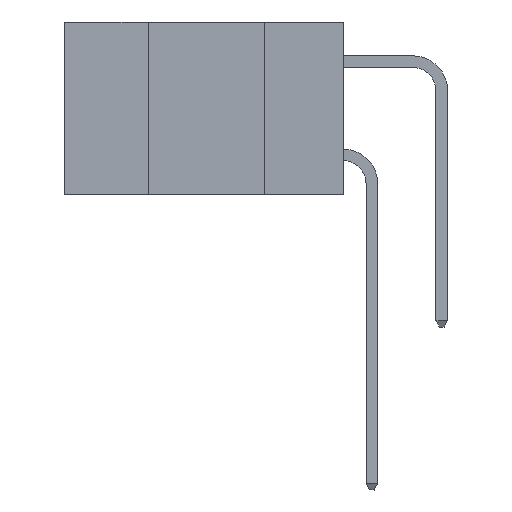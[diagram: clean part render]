
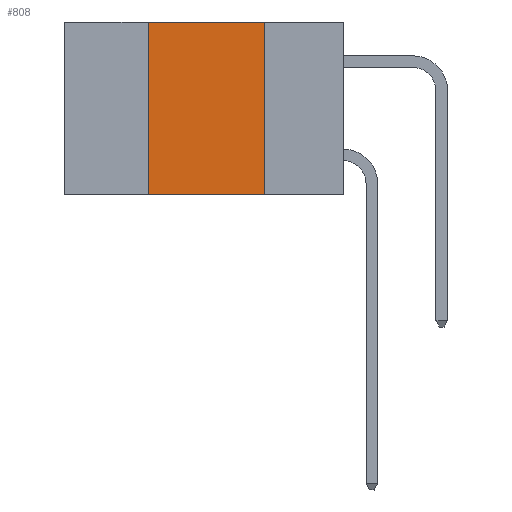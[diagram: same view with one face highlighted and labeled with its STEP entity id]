
A CAD part, left-side view. The second image highlights one B-rep face of the part: STEP entity #808.
In plain terms, the highlighted planar face has unit normal (-1, 0, 0).
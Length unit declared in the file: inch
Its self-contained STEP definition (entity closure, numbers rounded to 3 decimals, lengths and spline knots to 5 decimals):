
#54 = EDGE_CURVE ( 'NONE', #7547, #682, #2304, .T. ) ;
#215 = EDGE_CURVE ( 'NONE', #682, #5198, #5737, .T. ) ;
#250 = CARTESIAN_POINT ( 'NONE',  ( 0., 0.17, -0.37 ) ) ;
#503 = AXIS2_PLACEMENT_3D ( 'NONE', #5268, #9201, #7152 ) ;
#682 = VERTEX_POINT ( 'NONE', #9652 ) ;
#808 = ADVANCED_FACE ( 'NONE', ( #3222 ), #10155, .F. ) ;
#2027 = LINE ( 'NONE', #2223, #6362 ) ;
#2223 = CARTESIAN_POINT ( 'NONE',  ( 0., 0.6, -0.37 ) ) ;
#2249 = LINE ( 'NONE', #250, #9504 ) ;
#2304 = LINE ( 'NONE', #9115, #7276 ) ;
#3222 = FACE_OUTER_BOUND ( 'NONE', #10263, .T. ) ;
#3363 = VECTOR ( 'NONE', #8225, 39.37008 ) ;
#4380 = CARTESIAN_POINT ( 'NONE',  ( 0., 0.42, -0.37 ) ) ;
#4600 = ORIENTED_EDGE ( 'NONE', *, *, #11963, .T. ) ;
#4879 = DIRECTION ( 'NONE',  ( 0., 0., -1. ) ) ;
#5198 = VERTEX_POINT ( 'NONE', #9021 ) ;
#5268 = CARTESIAN_POINT ( 'NONE',  ( 0., 0.6, 0. ) ) ;
#5737 = LINE ( 'NONE', #12546, #3363 ) ;
#6362 = VECTOR ( 'NONE', #11786, 39.37008 ) ;
#7152 = DIRECTION ( 'NONE',  ( 0., 0., -1. ) ) ;
#7207 = CARTESIAN_POINT ( 'NONE',  ( 0., 0.17, -0.37 ) ) ;
#7276 = VECTOR ( 'NONE', #9889, 39.37008 ) ;
#7547 = VERTEX_POINT ( 'NONE', #4380 ) ;
#8225 = DIRECTION ( 'NONE',  ( 0., -1., 0. ) ) ;
#9021 = CARTESIAN_POINT ( 'NONE',  ( 0., 0.17, 0. ) ) ;
#9115 = CARTESIAN_POINT ( 'NONE',  ( 0., 0.42, -0.37 ) ) ;
#9201 = DIRECTION ( 'NONE',  ( 1., 0., 0. ) ) ;
#9504 = VECTOR ( 'NONE', #4879, 39.37008 ) ;
#9542 = EDGE_CURVE ( 'NONE', #5198, #10416, #2249, .T. ) ;
#9652 = CARTESIAN_POINT ( 'NONE',  ( 0., 0.42, 0. ) ) ;
#9889 = DIRECTION ( 'NONE',  ( 0., 0., 1. ) ) ;
#10155 = PLANE ( 'NONE',  #503 ) ;
#10157 = ORIENTED_EDGE ( 'NONE', *, *, #215, .F. ) ;
#10263 = EDGE_LOOP ( 'NONE', ( #10680, #10157, #11693, #4600 ) ) ;
#10416 = VERTEX_POINT ( 'NONE', #7207 ) ;
#10680 = ORIENTED_EDGE ( 'NONE', *, *, #9542, .F. ) ;
#11693 = ORIENTED_EDGE ( 'NONE', *, *, #54, .F. ) ;
#11786 = DIRECTION ( 'NONE',  ( 0., -1., 0. ) ) ;
#11963 = EDGE_CURVE ( 'NONE', #7547, #10416, #2027, .T. ) ;
#12546 = CARTESIAN_POINT ( 'NONE',  ( 0., 0.6, 0. ) ) ;
